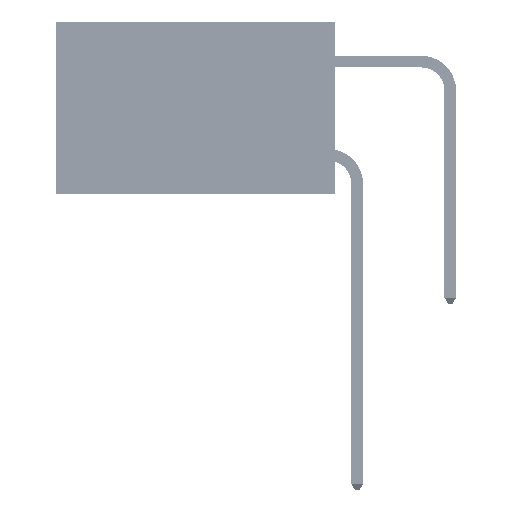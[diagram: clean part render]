
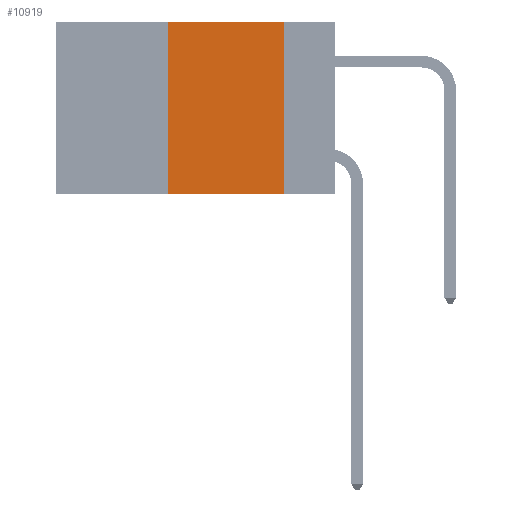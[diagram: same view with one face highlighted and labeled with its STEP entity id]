
A CAD part, left-side view. The second image highlights one B-rep face of the part: STEP entity #10919.
In plain terms, the highlighted planar face has unit normal (-1, 0, 0).
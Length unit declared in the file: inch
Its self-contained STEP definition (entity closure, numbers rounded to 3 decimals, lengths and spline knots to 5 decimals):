
#978 = AXIS2_PLACEMENT_3D ( 'NONE', #8920, #46254, #8365 ) ;
#2955 = DIRECTION ( 'NONE',  ( 0., -1., 0. ) ) ;
#3734 = CARTESIAN_POINT ( 'NONE',  ( 0., 0.36, -0.37 ) ) ;
#4071 = VERTEX_POINT ( 'NONE', #9856 ) ;
#4485 = CARTESIAN_POINT ( 'NONE',  ( 0., 0.6, 0. ) ) ;
#5041 = VERTEX_POINT ( 'NONE', #3734 ) ;
#7936 = CARTESIAN_POINT ( 'NONE',  ( 0., 0.36, 0. ) ) ;
#8365 = DIRECTION ( 'NONE',  ( 0., 0., -1. ) ) ;
#8467 = VERTEX_POINT ( 'NONE', #7936 ) ;
#8920 = CARTESIAN_POINT ( 'NONE',  ( 0., 0.6, 0. ) ) ;
#9856 = CARTESIAN_POINT ( 'NONE',  ( 0., 0.11, 0. ) ) ;
#9869 = LINE ( 'NONE', #4485, #26659 ) ;
#10919 = ADVANCED_FACE ( 'NONE', ( #42652 ), #20850, .F. ) ;
#12481 = CARTESIAN_POINT ( 'NONE',  ( 0., 0.11, -0.37 ) ) ;
#12848 = VECTOR ( 'NONE', #14548, 39.37008 ) ;
#14376 = CARTESIAN_POINT ( 'NONE',  ( 0., 0.36, 0. ) ) ;
#14548 = DIRECTION ( 'NONE',  ( 0., 0., 1. ) ) ;
#15297 = VECTOR ( 'NONE', #17755, 39.37008 ) ;
#15408 = EDGE_LOOP ( 'NONE', ( #33115, #32180, #27142, #34017 ) ) ;
#17755 = DIRECTION ( 'NONE',  ( 0., 0., -1. ) ) ;
#20584 = VERTEX_POINT ( 'NONE', #12481 ) ;
#20850 = PLANE ( 'NONE',  #978 ) ;
#26119 = EDGE_CURVE ( 'NONE', #5041, #8467, #41434, .T. ) ;
#26659 = VECTOR ( 'NONE', #33472, 39.37008 ) ;
#27142 = ORIENTED_EDGE ( 'NONE', *, *, #26119, .F. ) ;
#27720 = CARTESIAN_POINT ( 'NONE',  ( 0., 0.6, -0.37 ) ) ;
#32180 = ORIENTED_EDGE ( 'NONE', *, *, #35860, .F. ) ;
#33115 = ORIENTED_EDGE ( 'NONE', *, *, #40283, .F. ) ;
#33472 = DIRECTION ( 'NONE',  ( 0., -1., 0. ) ) ;
#34017 = ORIENTED_EDGE ( 'NONE', *, *, #50238, .T. ) ;
#35860 = EDGE_CURVE ( 'NONE', #8467, #4071, #9869, .T. ) ;
#36110 = VECTOR ( 'NONE', #2955, 39.37008 ) ;
#38718 = LINE ( 'NONE', #27720, #36110 ) ;
#40283 = EDGE_CURVE ( 'NONE', #4071, #20584, #46482, .T. ) ;
#41434 = LINE ( 'NONE', #14376, #12848 ) ;
#42652 = FACE_OUTER_BOUND ( 'NONE', #15408, .T. ) ;
#42790 = CARTESIAN_POINT ( 'NONE',  ( 0., 0.11, 0. ) ) ;
#46254 = DIRECTION ( 'NONE',  ( 1., 0., 0. ) ) ;
#46482 = LINE ( 'NONE', #42790, #15297 ) ;
#50238 = EDGE_CURVE ( 'NONE', #5041, #20584, #38718, .T. ) ;
